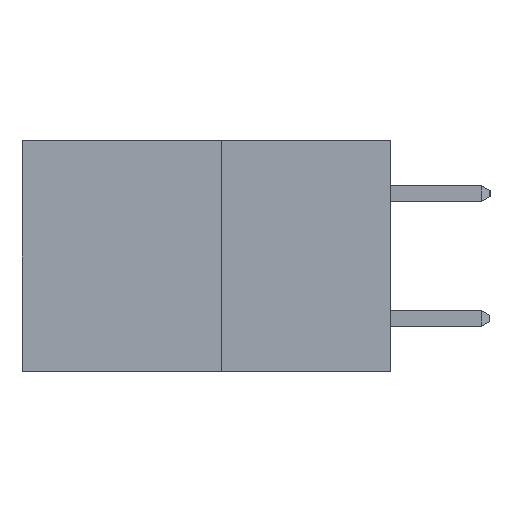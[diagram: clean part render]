
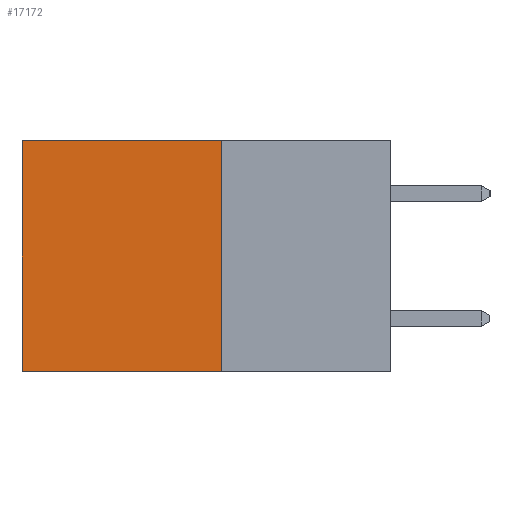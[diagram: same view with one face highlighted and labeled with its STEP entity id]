
A CAD part, left-side view. The second image highlights one B-rep face of the part: STEP entity #17172.
In plain terms, the highlighted planar face has unit normal (-1, 0, 0).
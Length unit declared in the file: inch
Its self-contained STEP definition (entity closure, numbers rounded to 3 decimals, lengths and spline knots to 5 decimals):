
#1118 = CARTESIAN_POINT ( 'NONE',  ( 0.277, 0.27, -0.37 ) ) ;
#1200 = VECTOR ( 'NONE', #19203, 39.37008 ) ;
#1237 = LINE ( 'NONE', #12594, #13604 ) ;
#1350 = EDGE_LOOP ( 'NONE', ( #21960, #6730, #6592, #15714 ) ) ;
#2655 = CARTESIAN_POINT ( 'NONE',  ( 0.277, 0.27, 0. ) ) ;
#3244 = DIRECTION ( 'NONE',  ( 0., 0., -1. ) ) ;
#3732 = VECTOR ( 'NONE', #4963, 39.37008 ) ;
#4963 = DIRECTION ( 'NONE',  ( 0., 1., 0. ) ) ;
#5790 = DIRECTION ( 'NONE',  ( 0., 0., -1. ) ) ;
#6592 = ORIENTED_EDGE ( 'NONE', *, *, #29157, .F. ) ;
#6730 = ORIENTED_EDGE ( 'NONE', *, *, #23234, .F. ) ;
#7299 = CARTESIAN_POINT ( 'NONE',  ( 0.277, 0.27, -0.37 ) ) ;
#7568 = CARTESIAN_POINT ( 'NONE',  ( 0.277, 0.59, -0.37 ) ) ;
#8362 = VERTEX_POINT ( 'NONE', #7299 ) ;
#9269 = CARTESIAN_POINT ( 'NONE',  ( 0.277, 0.59, -0.37 ) ) ;
#9626 = FACE_OUTER_BOUND ( 'NONE', #1350, .T. ) ;
#9914 = DIRECTION ( 'NONE',  ( 0., 0., -1. ) ) ;
#10091 = CARTESIAN_POINT ( 'NONE',  ( 0.277, 0.27, -0.37 ) ) ;
#11622 = LINE ( 'NONE', #7568, #28998 ) ;
#12594 = CARTESIAN_POINT ( 'NONE',  ( 0.277, 0.27, -0.37 ) ) ;
#12713 = VERTEX_POINT ( 'NONE', #24910 ) ;
#13604 = VECTOR ( 'NONE', #3244, 39.37008 ) ;
#14609 = CARTESIAN_POINT ( 'NONE',  ( 0.277, 0.59, 0. ) ) ;
#14992 = PLANE ( 'NONE',  #28359 ) ;
#15714 = ORIENTED_EDGE ( 'NONE', *, *, #23752, .T. ) ;
#16030 = LINE ( 'NONE', #2655, #3732 ) ;
#17172 = ADVANCED_FACE ( 'NONE', ( #9626 ), #14992, .F. ) ;
#18902 = LINE ( 'NONE', #10091, #1200 ) ;
#19203 = DIRECTION ( 'NONE',  ( 0., 1., 0. ) ) ;
#19588 = DIRECTION ( 'NONE',  ( 1., 0., 0. ) ) ;
#21732 = VERTEX_POINT ( 'NONE', #9269 ) ;
#21960 = ORIENTED_EDGE ( 'NONE', *, *, #25268, .T. ) ;
#23234 = EDGE_CURVE ( 'NONE', #8362, #21732, #18902, .T. ) ;
#23752 = EDGE_CURVE ( 'NONE', #12713, #28388, #16030, .T. ) ;
#24910 = CARTESIAN_POINT ( 'NONE',  ( 0.277, 0.27, 0. ) ) ;
#25268 = EDGE_CURVE ( 'NONE', #28388, #21732, #11622, .T. ) ;
#28359 = AXIS2_PLACEMENT_3D ( 'NONE', #1118, #19588, #5790 ) ;
#28388 = VERTEX_POINT ( 'NONE', #14609 ) ;
#28998 = VECTOR ( 'NONE', #9914, 39.37008 ) ;
#29157 = EDGE_CURVE ( 'NONE', #12713, #8362, #1237, .T. ) ;
